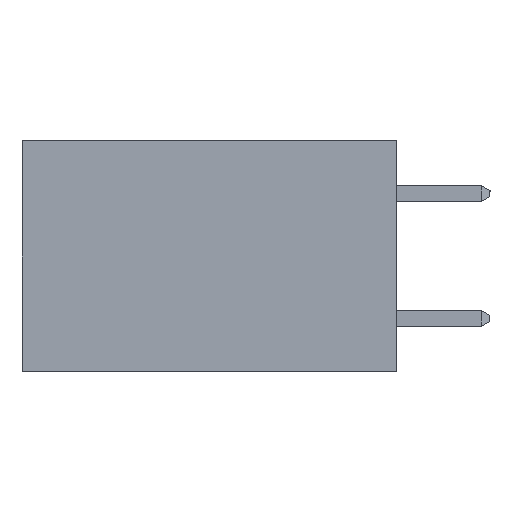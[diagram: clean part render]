
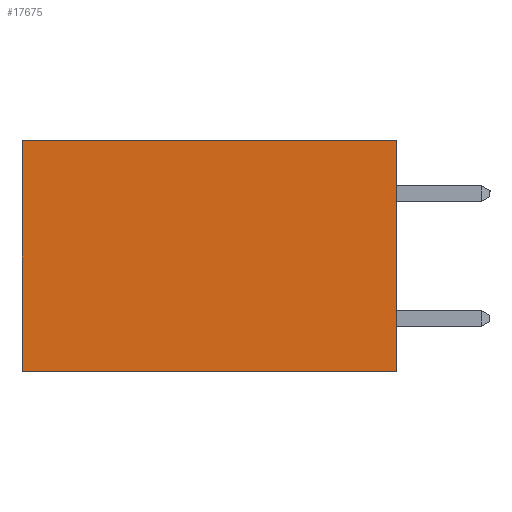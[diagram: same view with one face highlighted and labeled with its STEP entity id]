
A CAD part, left-side view. The second image highlights one B-rep face of the part: STEP entity #17675.
In plain terms, the highlighted planar face has unit normal (-1, 0, 0).
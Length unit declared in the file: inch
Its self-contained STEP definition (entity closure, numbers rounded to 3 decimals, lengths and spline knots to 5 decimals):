
#1445 = DIRECTION ( 'NONE',  ( 0., 1., 0. ) ) ;
#1766 = ORIENTED_EDGE ( 'NONE', *, *, #9135, .F. ) ;
#2064 = EDGE_CURVE ( 'NONE', #14036, #3868, #22360, .T. ) ;
#3375 = ORIENTED_EDGE ( 'NONE', *, *, #17232, .T. ) ;
#3868 = VERTEX_POINT ( 'NONE', #17974 ) ;
#4917 = DIRECTION ( 'NONE',  ( 0., 0., -1. ) ) ;
#5200 = DIRECTION ( 'NONE',  ( 0., 0., -1. ) ) ;
#5241 = ORIENTED_EDGE ( 'NONE', *, *, #2064, .T. ) ;
#6194 = AXIS2_PLACEMENT_3D ( 'NONE', #11567, #15775, #9531 ) ;
#6308 = VERTEX_POINT ( 'NONE', #15445 ) ;
#6644 = EDGE_LOOP ( 'NONE', ( #3375, #19141, #1766, #5241 ) ) ;
#6938 = VERTEX_POINT ( 'NONE', #16002 ) ;
#7068 = FACE_OUTER_BOUND ( 'NONE', #6644, .T. ) ;
#7497 = LINE ( 'NONE', #9561, #26097 ) ;
#9102 = EDGE_CURVE ( 'NONE', #6308, #6938, #9428, .T. ) ;
#9135 = EDGE_CURVE ( 'NONE', #14036, #6308, #15260, .T. ) ;
#9428 = LINE ( 'NONE', #17716, #25114 ) ;
#9531 = DIRECTION ( 'NONE',  ( 0., 0., -1. ) ) ;
#9561 = CARTESIAN_POINT ( 'NONE',  ( 0.2615, 0.6, -0.37 ) ) ;
#11567 = CARTESIAN_POINT ( 'NONE',  ( 0.2615, 0., -0.37 ) ) ;
#13782 = DIRECTION ( 'NONE',  ( 0., 1., 0. ) ) ;
#14036 = VERTEX_POINT ( 'NONE', #25987 ) ;
#15260 = LINE ( 'NONE', #23522, #17806 ) ;
#15445 = CARTESIAN_POINT ( 'NONE',  ( 0.2615, 0., -0.37 ) ) ;
#15775 = DIRECTION ( 'NONE',  ( 1., 0., 0. ) ) ;
#16002 = CARTESIAN_POINT ( 'NONE',  ( 0.2615, 0.6, -0.37 ) ) ;
#17232 = EDGE_CURVE ( 'NONE', #3868, #6938, #7497, .T. ) ;
#17675 = ADVANCED_FACE ( 'NONE', ( #7068 ), #26181, .F. ) ;
#17716 = CARTESIAN_POINT ( 'NONE',  ( 0.2615, 0., -0.37 ) ) ;
#17806 = VECTOR ( 'NONE', #4917, 39.37008 ) ;
#17974 = CARTESIAN_POINT ( 'NONE',  ( 0.2615, 0.6, 0. ) ) ;
#19141 = ORIENTED_EDGE ( 'NONE', *, *, #9102, .F. ) ;
#22279 = VECTOR ( 'NONE', #1445, 39.37008 ) ;
#22360 = LINE ( 'NONE', #26136, #22279 ) ;
#23522 = CARTESIAN_POINT ( 'NONE',  ( 0.2615, 0., -0.37 ) ) ;
#25114 = VECTOR ( 'NONE', #13782, 39.37008 ) ;
#25987 = CARTESIAN_POINT ( 'NONE',  ( 0.2615, 0., 0. ) ) ;
#26097 = VECTOR ( 'NONE', #5200, 39.37008 ) ;
#26136 = CARTESIAN_POINT ( 'NONE',  ( 0.2615, 0., 0. ) ) ;
#26181 = PLANE ( 'NONE',  #6194 ) ;
